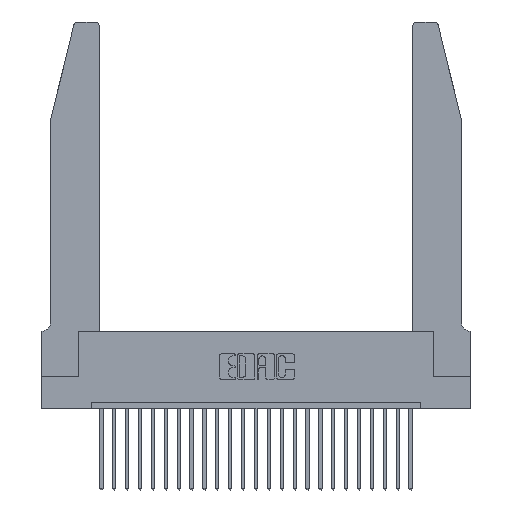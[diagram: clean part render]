
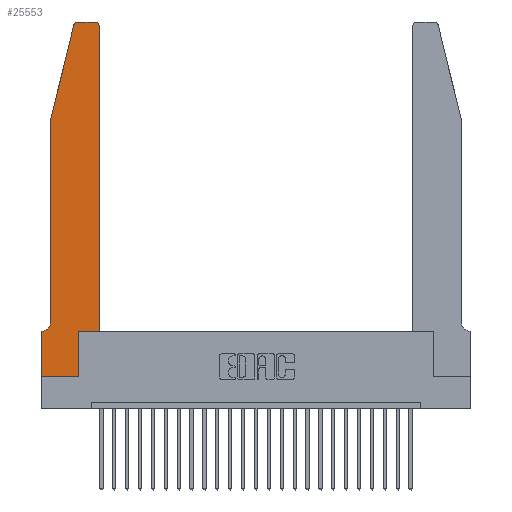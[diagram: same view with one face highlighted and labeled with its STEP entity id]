
A CAD part, top view. The second image highlights one B-rep face of the part: STEP entity #25553.
In plain terms, the highlighted planar face has unit normal (0, 0, 1).
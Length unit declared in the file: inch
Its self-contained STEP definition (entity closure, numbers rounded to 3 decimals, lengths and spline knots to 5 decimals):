
#427 = CARTESIAN_POINT ( 'NONE',  ( 0., 0.35, 0.37 ) ) ;
#561 = CARTESIAN_POINT ( 'NONE',  ( 0.4205, 2.72, 0.37 ) ) ;
#593 = VECTOR ( 'NONE', #5524, 39.37008 ) ;
#772 = EDGE_CURVE ( 'NONE', #19308, #7519, #1423, .T. ) ;
#1105 = VERTEX_POINT ( 'NONE', #13975 ) ;
#1129 = ORIENTED_EDGE ( 'NONE', *, *, #22636, .T. ) ;
#1271 = EDGE_CURVE ( 'NONE', #8122, #23580, #13603, .T. ) ;
#1423 = LINE ( 'NONE', #10451, #17687 ) ;
#1507 = AXIS2_PLACEMENT_3D ( 'NONE', #2143, #21831, #22187 ) ;
#1598 = CARTESIAN_POINT ( 'NONE',  ( 0., 0., 0.37 ) ) ;
#1985 = VECTOR ( 'NONE', #5610, 39.37008 ) ;
#1988 = ORIENTED_EDGE ( 'NONE', *, *, #3436, .T. ) ;
#2143 = CARTESIAN_POINT ( 'NONE',  ( 0.0055, 0.42, 0.37 ) ) ;
#2467 = VERTEX_POINT ( 'NONE', #10926 ) ;
#2853 = LINE ( 'NONE', #23364, #16916 ) ;
#2867 = VERTEX_POINT ( 'NONE', #4648 ) ;
#3074 = CARTESIAN_POINT ( 'NONE',  ( 0.284, 2.75, 0.37 ) ) ;
#3121 = LINE ( 'NONE', #9377, #593 ) ;
#3242 = DIRECTION ( 'NONE',  ( 0., 1., 0. ) ) ;
#3436 = EDGE_CURVE ( 'NONE', #12595, #2867, #2853, .T. ) ;
#3488 = ORIENTED_EDGE ( 'NONE', *, *, #17122, .T. ) ;
#3632 = ORIENTED_EDGE ( 'NONE', *, *, #10276, .T. ) ;
#3687 = DIRECTION ( 'NONE',  ( 1., 0., 0. ) ) ;
#3774 = AXIS2_PLACEMENT_3D ( 'NONE', #13637, #15650, #3687 ) ;
#4057 = CARTESIAN_POINT ( 'NONE',  ( 0.4505, 0.35, 0.37 ) ) ;
#4471 = CARTESIAN_POINT ( 'NONE',  ( 0.0055, 0.35, 0.37 ) ) ;
#4648 = CARTESIAN_POINT ( 'NONE',  ( 0.2865, 0.35, 0.37 ) ) ;
#4995 = CIRCLE ( 'NONE', #23961, 0.03 ) ;
#5524 = DIRECTION ( 'NONE',  ( 1., 0., 0. ) ) ;
#5568 = CARTESIAN_POINT ( 'NONE',  ( 0.2865, 0., 0.37 ) ) ;
#5610 = DIRECTION ( 'NONE',  ( -1., 0., 0. ) ) ;
#5966 = VERTEX_POINT ( 'NONE', #3074 ) ;
#5976 = CARTESIAN_POINT ( 'NONE',  ( 0., 0., 0.37 ) ) ;
#6005 = FACE_OUTER_BOUND ( 'NONE', #7533, .T. ) ;
#6184 = LINE ( 'NONE', #14931, #22053 ) ;
#6399 = ORIENTED_EDGE ( 'NONE', *, *, #20374, .T. ) ;
#6642 = DIRECTION ( 'NONE',  ( 0., 0., 1. ) ) ;
#7362 = VECTOR ( 'NONE', #24529, 39.37008 ) ;
#7519 = VERTEX_POINT ( 'NONE', #15205 ) ;
#7533 = EDGE_LOOP ( 'NONE', ( #3488, #6399, #17241, #10837, #1129, #8894, #9612, #3632, #1988, #16519, #13199, #7852 ) ) ;
#7852 = ORIENTED_EDGE ( 'NONE', *, *, #13930, .T. ) ;
#8055 = DIRECTION ( 'NONE',  ( 1., 0., 0. ) ) ;
#8122 = VERTEX_POINT ( 'NONE', #4057 ) ;
#8894 = ORIENTED_EDGE ( 'NONE', *, *, #14923, .T. ) ;
#9377 = CARTESIAN_POINT ( 'NONE',  ( 0.4505, 0.35, 0.37 ) ) ;
#9612 = ORIENTED_EDGE ( 'NONE', *, *, #10977, .T. ) ;
#9895 = AXIS2_PLACEMENT_3D ( 'NONE', #22648, #10832, #10739 ) ;
#10231 = LINE ( 'NONE', #5976, #23617 ) ;
#10276 = EDGE_CURVE ( 'NONE', #2467, #12595, #10231, .T. ) ;
#10446 = CARTESIAN_POINT ( 'NONE',  ( 0.25487, 2.72718, 0.37 ) ) ;
#10451 = CARTESIAN_POINT ( 'NONE',  ( 0.0755, 2., 0.37 ) ) ;
#10502 = LINE ( 'NONE', #1598, #22963 ) ;
#10739 = DIRECTION ( 'NONE',  ( 1., 0., 0. ) ) ;
#10832 = DIRECTION ( 'NONE',  ( 0., 0., 1. ) ) ;
#10837 = ORIENTED_EDGE ( 'NONE', *, *, #25042, .T. ) ;
#10915 = VERTEX_POINT ( 'NONE', #4471 ) ;
#10926 = CARTESIAN_POINT ( 'NONE',  ( 0., 0., 0.37 ) ) ;
#10977 = EDGE_CURVE ( 'NONE', #25115, #2467, #10502, .T. ) ;
#10991 = CARTESIAN_POINT ( 'NONE',  ( 0.0755, 0.42, 0.37 ) ) ;
#11525 = CARTESIAN_POINT ( 'NONE',  ( 0.2605, 2.75, 0.37 ) ) ;
#11535 = PLANE ( 'NONE',  #3774 ) ;
#11759 = DIRECTION ( 'NONE',  ( 0., -1., 0. ) ) ;
#12595 = VERTEX_POINT ( 'NONE', #5568 ) ;
#13199 = ORIENTED_EDGE ( 'NONE', *, *, #1271, .T. ) ;
#13603 = LINE ( 'NONE', #22414, #7362 ) ;
#13637 = CARTESIAN_POINT ( 'NONE',  ( 0., 0.35, 0.37 ) ) ;
#13930 = EDGE_CURVE ( 'NONE', #23580, #1105, #4995, .T. ) ;
#13975 = CARTESIAN_POINT ( 'NONE',  ( 0.4205, 2.75, 0.37 ) ) ;
#14617 = CIRCLE ( 'NONE', #1507, 0.07 ) ;
#14923 = EDGE_CURVE ( 'NONE', #10915, #25115, #6184, .T. ) ;
#14931 = CARTESIAN_POINT ( 'NONE',  ( 0.0755, 0.35, 0.37 ) ) ;
#15205 = CARTESIAN_POINT ( 'NONE',  ( 0.0755, 2., 0.37 ) ) ;
#15650 = DIRECTION ( 'NONE',  ( 0., 0., 1. ) ) ;
#16519 = ORIENTED_EDGE ( 'NONE', *, *, #21223, .T. ) ;
#16916 = VECTOR ( 'NONE', #3242, 39.37008 ) ;
#17122 = EDGE_CURVE ( 'NONE', #1105, #5966, #19794, .T. ) ;
#17228 = VECTOR ( 'NONE', #18028, 39.37008 ) ;
#17241 = ORIENTED_EDGE ( 'NONE', *, *, #772, .T. ) ;
#17319 = VERTEX_POINT ( 'NONE', #10991 ) ;
#17687 = VECTOR ( 'NONE', #24372, 39.37008 ) ;
#18028 = DIRECTION ( 'NONE',  ( 0., -1., 0. ) ) ;
#18152 = LINE ( 'NONE', #23913, #17228 ) ;
#18482 = CIRCLE ( 'NONE', #9895, 0.03 ) ;
#19308 = VERTEX_POINT ( 'NONE', #10446 ) ;
#19794 = LINE ( 'NONE', #11525, #1985 ) ;
#20374 = EDGE_CURVE ( 'NONE', #5966, #19308, #18482, .T. ) ;
#20556 = DIRECTION ( 'NONE',  ( 1., 0., 0. ) ) ;
#21223 = EDGE_CURVE ( 'NONE', #2867, #8122, #3121, .T. ) ;
#21831 = DIRECTION ( 'NONE',  ( 0., 0., -1. ) ) ;
#22053 = VECTOR ( 'NONE', #24748, 39.37008 ) ;
#22187 = DIRECTION ( 'NONE',  ( -1., 0., 0. ) ) ;
#22414 = CARTESIAN_POINT ( 'NONE',  ( 0.4505, 0.35, 0.37 ) ) ;
#22636 = EDGE_CURVE ( 'NONE', #17319, #10915, #14617, .T. ) ;
#22648 = CARTESIAN_POINT ( 'NONE',  ( 0.284, 2.72, 0.37 ) ) ;
#22963 = VECTOR ( 'NONE', #11759, 39.37008 ) ;
#23364 = CARTESIAN_POINT ( 'NONE',  ( 0.2865, 0.35, 0.37 ) ) ;
#23580 = VERTEX_POINT ( 'NONE', #25132 ) ;
#23617 = VECTOR ( 'NONE', #8055, 39.37008 ) ;
#23913 = CARTESIAN_POINT ( 'NONE',  ( 0.0755, 2., 0.37 ) ) ;
#23961 = AXIS2_PLACEMENT_3D ( 'NONE', #561, #6642, #20556 ) ;
#24372 = DIRECTION ( 'NONE',  ( -0.239, -0.971, 0. ) ) ;
#24529 = DIRECTION ( 'NONE',  ( 0., 1., 0. ) ) ;
#24748 = DIRECTION ( 'NONE',  ( -1., 0., 0. ) ) ;
#25042 = EDGE_CURVE ( 'NONE', #7519, #17319, #18152, .T. ) ;
#25115 = VERTEX_POINT ( 'NONE', #427 ) ;
#25132 = CARTESIAN_POINT ( 'NONE',  ( 0.4505, 2.72, 0.37 ) ) ;
#25553 = ADVANCED_FACE ( 'NONE', ( #6005 ), #11535, .T. ) ;
